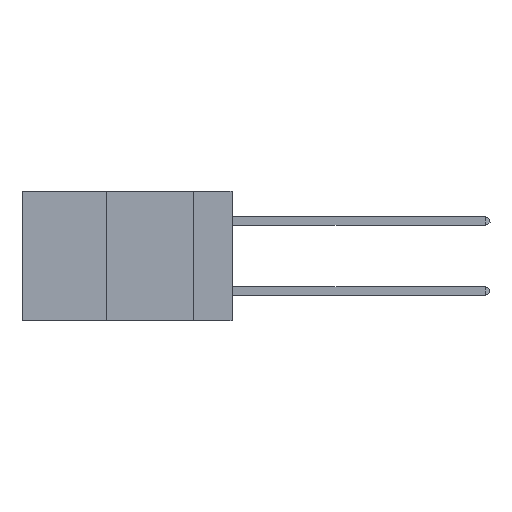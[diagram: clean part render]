
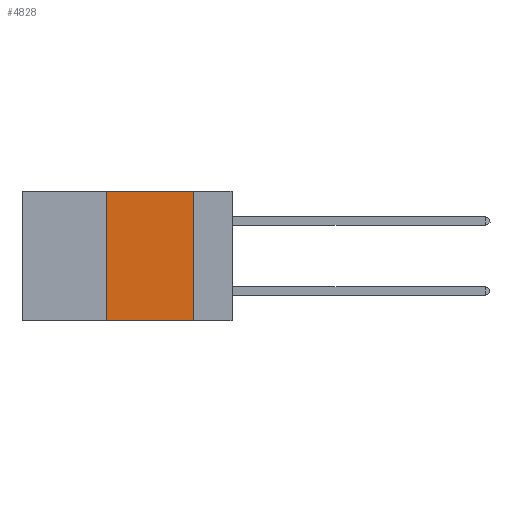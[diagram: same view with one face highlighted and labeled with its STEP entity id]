
A CAD part, left-side view. The second image highlights one B-rep face of the part: STEP entity #4828.
In plain terms, the highlighted planar face has unit normal (-1, 0, 0).
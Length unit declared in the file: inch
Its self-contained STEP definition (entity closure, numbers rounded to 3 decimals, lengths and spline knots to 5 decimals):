
#4 = VECTOR ( 'NONE', #9416, 39.37008 ) ;
#1087 = CARTESIAN_POINT ( 'NONE',  ( 0., 0.36, -0.37 ) ) ;
#1230 = CARTESIAN_POINT ( 'NONE',  ( 0., 0.36, 0. ) ) ;
#1893 = DIRECTION ( 'NONE',  ( 0., 0., -1. ) ) ;
#2445 = VECTOR ( 'NONE', #14923, 39.37008 ) ;
#2932 = LINE ( 'NONE', #15194, #4 ) ;
#3043 = ORIENTED_EDGE ( 'NONE', *, *, #13749, .F. ) ;
#4828 = ADVANCED_FACE ( 'NONE', ( #11541 ), #13886, .F. ) ;
#4919 = CARTESIAN_POINT ( 'NONE',  ( 0., 0.11, 0. ) ) ;
#4941 = DIRECTION ( 'NONE',  ( 0., -1., 0. ) ) ;
#5328 = CARTESIAN_POINT ( 'NONE',  ( 0., 0.6, 0. ) ) ;
#5583 = CARTESIAN_POINT ( 'NONE',  ( 0., 0.11, 0. ) ) ;
#6233 = LINE ( 'NONE', #4919, #2445 ) ;
#6293 = CARTESIAN_POINT ( 'NONE',  ( 0., 0.6, 0. ) ) ;
#6426 = LINE ( 'NONE', #1230, #16071 ) ;
#7248 = ORIENTED_EDGE ( 'NONE', *, *, #16956, .F. ) ;
#7494 = VERTEX_POINT ( 'NONE', #5583 ) ;
#8284 = DIRECTION ( 'NONE',  ( 0., 0., 1. ) ) ;
#8504 = EDGE_CURVE ( 'NONE', #12896, #11228, #6426, .T. ) ;
#8845 = CARTESIAN_POINT ( 'NONE',  ( 0., 0.36, 0. ) ) ;
#9416 = DIRECTION ( 'NONE',  ( 0., -1., 0. ) ) ;
#9571 = DIRECTION ( 'NONE',  ( 1., 0., 0. ) ) ;
#9808 = VECTOR ( 'NONE', #4941, 39.37008 ) ;
#10159 = AXIS2_PLACEMENT_3D ( 'NONE', #5328, #9571, #1893 ) ;
#10217 = VERTEX_POINT ( 'NONE', #14263 ) ;
#11228 = VERTEX_POINT ( 'NONE', #8845 ) ;
#11541 = FACE_OUTER_BOUND ( 'NONE', #14265, .T. ) ;
#12896 = VERTEX_POINT ( 'NONE', #1087 ) ;
#13749 = EDGE_CURVE ( 'NONE', #11228, #7494, #15192, .T. ) ;
#13886 = PLANE ( 'NONE',  #10159 ) ;
#14263 = CARTESIAN_POINT ( 'NONE',  ( 0., 0.11, -0.37 ) ) ;
#14265 = EDGE_LOOP ( 'NONE', ( #7248, #3043, #14554, #18092 ) ) ;
#14554 = ORIENTED_EDGE ( 'NONE', *, *, #8504, .F. ) ;
#14923 = DIRECTION ( 'NONE',  ( 0., 0., -1. ) ) ;
#15133 = EDGE_CURVE ( 'NONE', #12896, #10217, #2932, .T. ) ;
#15192 = LINE ( 'NONE', #6293, #9808 ) ;
#15194 = CARTESIAN_POINT ( 'NONE',  ( 0., 0.6, -0.37 ) ) ;
#16071 = VECTOR ( 'NONE', #8284, 39.37008 ) ;
#16956 = EDGE_CURVE ( 'NONE', #7494, #10217, #6233, .T. ) ;
#18092 = ORIENTED_EDGE ( 'NONE', *, *, #15133, .T. ) ;
